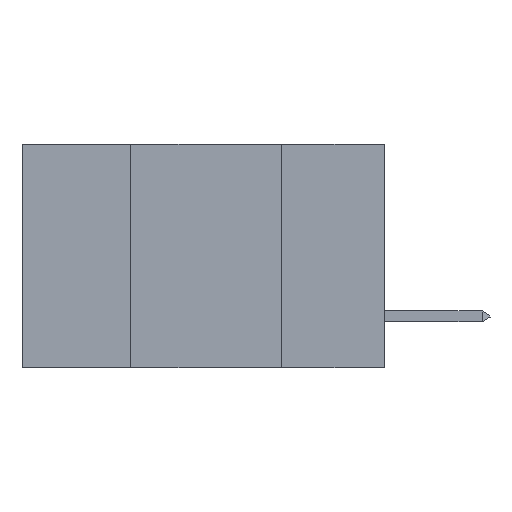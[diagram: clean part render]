
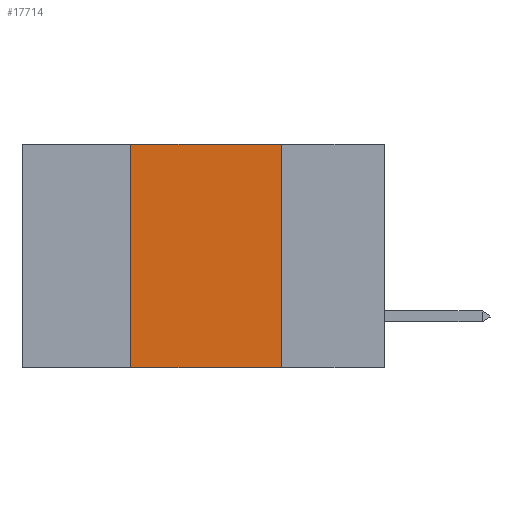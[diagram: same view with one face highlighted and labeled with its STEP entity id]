
A CAD part, left-side view. The second image highlights one B-rep face of the part: STEP entity #17714.
In plain terms, the highlighted planar face has unit normal (-1, 0, 0).
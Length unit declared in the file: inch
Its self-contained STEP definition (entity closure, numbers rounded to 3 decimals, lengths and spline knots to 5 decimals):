
#268 = AXIS2_PLACEMENT_3D ( 'NONE', #12994, #26707, #28794 ) ;
#826 = DIRECTION ( 'NONE',  ( 0., -1., 0. ) ) ;
#1130 = CARTESIAN_POINT ( 'NONE',  ( 0., 0.6, 0. ) ) ;
#2472 = VECTOR ( 'NONE', #16646, 39.37008 ) ;
#4172 = FACE_OUTER_BOUND ( 'NONE', #9325, .T. ) ;
#4193 = CARTESIAN_POINT ( 'NONE',  ( 0., 0.17, -0.37 ) ) ;
#4601 = DIRECTION ( 'NONE',  ( 0., 0., -1. ) ) ;
#5492 = CARTESIAN_POINT ( 'NONE',  ( 0., 0.42, 0. ) ) ;
#7160 = CARTESIAN_POINT ( 'NONE',  ( 0., 0.17, 0. ) ) ;
#7545 = VECTOR ( 'NONE', #826, 39.37008 ) ;
#9325 = EDGE_LOOP ( 'NONE', ( #22930, #16549, #28987, #22772 ) ) ;
#9908 = DIRECTION ( 'NONE',  ( 0., -1., 0. ) ) ;
#11039 = CARTESIAN_POINT ( 'NONE',  ( 0., 0.42, 0. ) ) ;
#11347 = VECTOR ( 'NONE', #4601, 39.37008 ) ;
#12762 = EDGE_CURVE ( 'NONE', #16339, #17112, #28380, .T. ) ;
#12994 = CARTESIAN_POINT ( 'NONE',  ( 0., 0.6, 0. ) ) ;
#13501 = VERTEX_POINT ( 'NONE', #4193 ) ;
#14259 = EDGE_CURVE ( 'NONE', #17112, #13501, #21945, .T. ) ;
#15213 = VERTEX_POINT ( 'NONE', #15790 ) ;
#15373 = PLANE ( 'NONE',  #268 ) ;
#15790 = CARTESIAN_POINT ( 'NONE',  ( 0., 0.42, -0.37 ) ) ;
#16003 = EDGE_CURVE ( 'NONE', #15213, #16339, #21248, .T. ) ;
#16154 = CARTESIAN_POINT ( 'NONE',  ( 0., 0.17, 0. ) ) ;
#16339 = VERTEX_POINT ( 'NONE', #11039 ) ;
#16549 = ORIENTED_EDGE ( 'NONE', *, *, #12762, .F. ) ;
#16646 = DIRECTION ( 'NONE',  ( 0., 0., 1. ) ) ;
#17112 = VERTEX_POINT ( 'NONE', #7160 ) ;
#17714 = ADVANCED_FACE ( 'NONE', ( #4172 ), #15373, .F. ) ;
#19158 = VECTOR ( 'NONE', #9908, 39.37008 ) ;
#21182 = EDGE_CURVE ( 'NONE', #15213, #13501, #22711, .T. ) ;
#21248 = LINE ( 'NONE', #5492, #2472 ) ;
#21945 = LINE ( 'NONE', #16154, #11347 ) ;
#22711 = LINE ( 'NONE', #23407, #19158 ) ;
#22772 = ORIENTED_EDGE ( 'NONE', *, *, #21182, .T. ) ;
#22930 = ORIENTED_EDGE ( 'NONE', *, *, #14259, .F. ) ;
#23407 = CARTESIAN_POINT ( 'NONE',  ( 0., 0.6, -0.37 ) ) ;
#26707 = DIRECTION ( 'NONE',  ( 1., 0., 0. ) ) ;
#28380 = LINE ( 'NONE', #1130, #7545 ) ;
#28794 = DIRECTION ( 'NONE',  ( 0., 0., -1. ) ) ;
#28987 = ORIENTED_EDGE ( 'NONE', *, *, #16003, .F. ) ;
